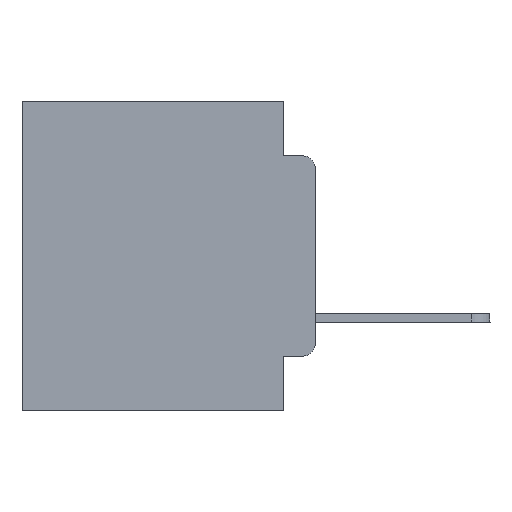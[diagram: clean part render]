
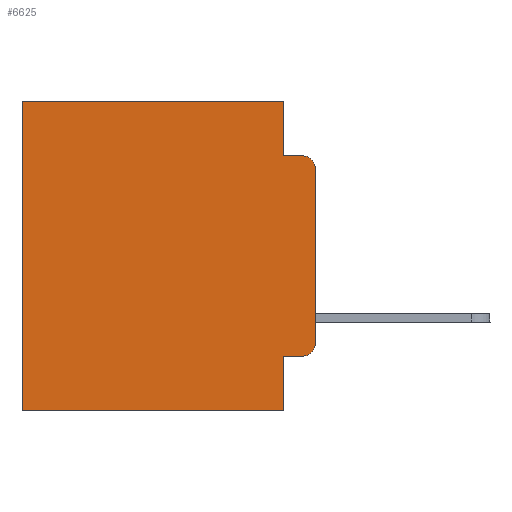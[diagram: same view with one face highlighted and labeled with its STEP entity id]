
A CAD part, left-side view. The second image highlights one B-rep face of the part: STEP entity #6625.
In plain terms, the highlighted planar face has unit normal (-1, 0, 0).
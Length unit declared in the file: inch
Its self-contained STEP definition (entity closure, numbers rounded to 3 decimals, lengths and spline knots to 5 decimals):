
#476 = VECTOR ( 'NONE', #2926, 39.37008 ) ;
#577 = VERTEX_POINT ( 'NONE', #26258 ) ;
#762 = EDGE_CURVE ( 'NONE', #17906, #24160, #21124, .T. ) ;
#1069 = ORIENTED_EDGE ( 'NONE', *, *, #15015, .F. ) ;
#1114 = EDGE_CURVE ( 'NONE', #10332, #577, #21736, .T. ) ;
#1133 = CARTESIAN_POINT ( 'NONE',  ( 0.298, 0., 0. ) ) ;
#1700 = DIRECTION ( 'NONE',  ( 0., 1., 0. ) ) ;
#1994 = EDGE_LOOP ( 'NONE', ( #14443, #5249, #25890, #8588, #4891, #19888, #10668, #1069, #6873, #6799 ) ) ;
#1997 = CIRCLE ( 'NONE', #5356, 0.02 ) ;
#2421 = VECTOR ( 'NONE', #12680, 39.37008 ) ;
#2564 = VERTEX_POINT ( 'NONE', #17104 ) ;
#2926 = DIRECTION ( 'NONE',  ( 0., 0., -1. ) ) ;
#3652 = EDGE_CURVE ( 'NONE', #17906, #10332, #21429, .T. ) ;
#3699 = VERTEX_POINT ( 'NONE', #19678 ) ;
#3710 = CARTESIAN_POINT ( 'NONE',  ( 0.298, 0.473, 0. ) ) ;
#4101 = VECTOR ( 'NONE', #5500, 39.37008 ) ;
#4581 = CIRCLE ( 'NONE', #18047, 0.02 ) ;
#4728 = VECTOR ( 'NONE', #5050, 39.37008 ) ;
#4891 = ORIENTED_EDGE ( 'NONE', *, *, #762, .T. ) ;
#5050 = DIRECTION ( 'NONE',  ( 0., -1., 0. ) ) ;
#5188 = DIRECTION ( 'NONE',  ( 0., 0., -1. ) ) ;
#5249 = ORIENTED_EDGE ( 'NONE', *, *, #27599, .T. ) ;
#5260 = CARTESIAN_POINT ( 'NONE',  ( 0.298, 0.473, 0. ) ) ;
#5338 = PLANE ( 'NONE',  #18936 ) ;
#5356 = AXIS2_PLACEMENT_3D ( 'NONE', #27190, #20902, #27288 ) ;
#5500 = DIRECTION ( 'NONE',  ( 0., 1., 0. ) ) ;
#5660 = LINE ( 'NONE', #20989, #10322 ) ;
#6625 = ADVANCED_FACE ( 'NONE', ( #7298 ), #5338, .F. ) ;
#6799 = ORIENTED_EDGE ( 'NONE', *, *, #26955, .T. ) ;
#6873 = ORIENTED_EDGE ( 'NONE', *, *, #11038, .T. ) ;
#7200 = CARTESIAN_POINT ( 'NONE',  ( 0.298, 0., -0.5 ) ) ;
#7298 = FACE_OUTER_BOUND ( 'NONE', #1994, .T. ) ;
#8588 = ORIENTED_EDGE ( 'NONE', *, *, #3652, .F. ) ;
#9105 = VECTOR ( 'NONE', #1700, 39.37008 ) ;
#9283 = CARTESIAN_POINT ( 'NONE',  ( 0.298, 0.02, -0.4115 ) ) ;
#9518 = EDGE_CURVE ( 'NONE', #2564, #24109, #16079, .T. ) ;
#10322 = VECTOR ( 'NONE', #14628, 39.37008 ) ;
#10332 = VERTEX_POINT ( 'NONE', #12068 ) ;
#10668 = ORIENTED_EDGE ( 'NONE', *, *, #9518, .F. ) ;
#11038 = EDGE_CURVE ( 'NONE', #3699, #12221, #5660, .T. ) ;
#11549 = CARTESIAN_POINT ( 'NONE',  ( 0.298, 0.051, 0. ) ) ;
#12068 = CARTESIAN_POINT ( 'NONE',  ( 0.298, 0.051, -0.0885 ) ) ;
#12221 = VERTEX_POINT ( 'NONE', #9283 ) ;
#12277 = CARTESIAN_POINT ( 'NONE',  ( 0.298, 0.02, -0.1085 ) ) ;
#12578 = CARTESIAN_POINT ( 'NONE',  ( 0.298, 0., 0. ) ) ;
#12680 = DIRECTION ( 'NONE',  ( 0., 0., -1. ) ) ;
#13689 = DIRECTION ( 'NONE',  ( 0., 0., -1. ) ) ;
#14395 = LINE ( 'NONE', #26677, #16731 ) ;
#14401 = DIRECTION ( 'NONE',  ( -1., 0., 0. ) ) ;
#14443 = ORIENTED_EDGE ( 'NONE', *, *, #15690, .F. ) ;
#14628 = DIRECTION ( 'NONE',  ( 0., -1., 0. ) ) ;
#14796 = LINE ( 'NONE', #17718, #476 ) ;
#15015 = EDGE_CURVE ( 'NONE', #3699, #2564, #14796, .T. ) ;
#15690 = EDGE_CURVE ( 'NONE', #16975, #24224, #14395, .T. ) ;
#16042 = VECTOR ( 'NONE', #20175, 39.37008 ) ;
#16079 = LINE ( 'NONE', #7200, #4101 ) ;
#16406 = CARTESIAN_POINT ( 'NONE',  ( 0.298, 0., -0.3915 ) ) ;
#16541 = EDGE_CURVE ( 'NONE', #24160, #24109, #21709, .T. ) ;
#16731 = VECTOR ( 'NONE', #5188, 39.37008 ) ;
#16975 = VERTEX_POINT ( 'NONE', #18650 ) ;
#17104 = CARTESIAN_POINT ( 'NONE',  ( 0.298, 0.051, -0.5 ) ) ;
#17718 = CARTESIAN_POINT ( 'NONE',  ( 0.298, 0.051, 0. ) ) ;
#17906 = VERTEX_POINT ( 'NONE', #11549 ) ;
#18047 = AXIS2_PLACEMENT_3D ( 'NONE', #12277, #14401, #23084 ) ;
#18650 = CARTESIAN_POINT ( 'NONE',  ( 0.298, 0., -0.1085 ) ) ;
#18936 = AXIS2_PLACEMENT_3D ( 'NONE', #1133, #26811, #13689 ) ;
#19678 = CARTESIAN_POINT ( 'NONE',  ( 0.298, 0.051, -0.4115 ) ) ;
#19888 = ORIENTED_EDGE ( 'NONE', *, *, #16541, .T. ) ;
#20175 = DIRECTION ( 'NONE',  ( 0., 0., -1. ) ) ;
#20902 = DIRECTION ( 'NONE',  ( -1., 0., 0. ) ) ;
#20989 = CARTESIAN_POINT ( 'NONE',  ( 0.298, 0.051, -0.4115 ) ) ;
#21124 = LINE ( 'NONE', #12578, #9105 ) ;
#21429 = LINE ( 'NONE', #25467, #2421 ) ;
#21709 = LINE ( 'NONE', #5260, #16042 ) ;
#21736 = LINE ( 'NONE', #26539, #4728 ) ;
#23084 = DIRECTION ( 'NONE',  ( 0., 0., -1. ) ) ;
#24109 = VERTEX_POINT ( 'NONE', #24951 ) ;
#24160 = VERTEX_POINT ( 'NONE', #3710 ) ;
#24224 = VERTEX_POINT ( 'NONE', #16406 ) ;
#24951 = CARTESIAN_POINT ( 'NONE',  ( 0.298, 0.473, -0.5 ) ) ;
#25467 = CARTESIAN_POINT ( 'NONE',  ( 0.298, 0.051, 0. ) ) ;
#25890 = ORIENTED_EDGE ( 'NONE', *, *, #1114, .F. ) ;
#26258 = CARTESIAN_POINT ( 'NONE',  ( 0.298, 0.02, -0.0885 ) ) ;
#26539 = CARTESIAN_POINT ( 'NONE',  ( 0.298, 0.051, -0.0885 ) ) ;
#26677 = CARTESIAN_POINT ( 'NONE',  ( 0.298, 0., 0. ) ) ;
#26811 = DIRECTION ( 'NONE',  ( 1., 0., 0. ) ) ;
#26955 = EDGE_CURVE ( 'NONE', #12221, #24224, #1997, .T. ) ;
#27190 = CARTESIAN_POINT ( 'NONE',  ( 0.298, 0.02, -0.3915 ) ) ;
#27288 = DIRECTION ( 'NONE',  ( 0., 0., -1. ) ) ;
#27599 = EDGE_CURVE ( 'NONE', #16975, #577, #4581, .T. ) ;
